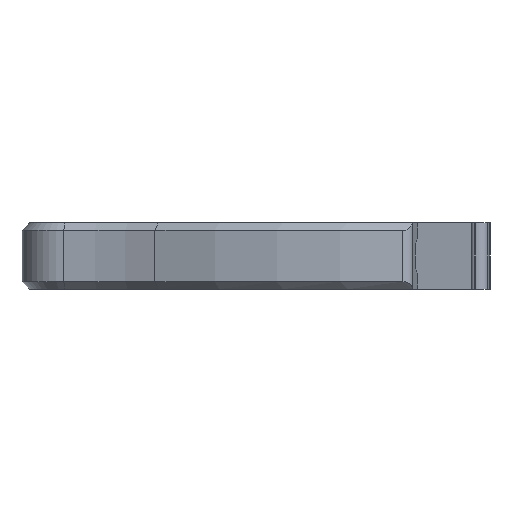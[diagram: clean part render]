
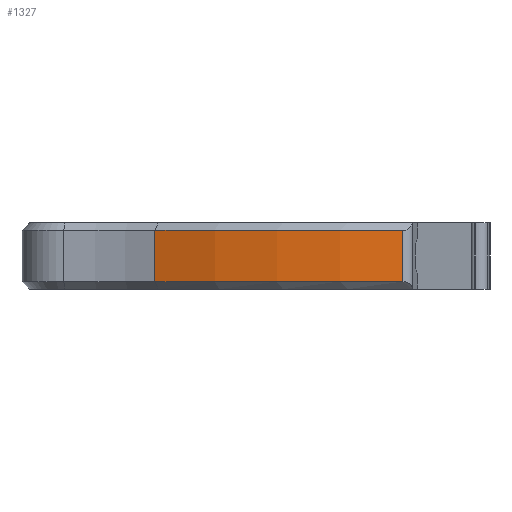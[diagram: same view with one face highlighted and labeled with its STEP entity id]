
A CAD part, left-side view. The second image highlights one B-rep face of the part: STEP entity #1327.
In plain terms, the highlighted cylindrical face has radius 77.47 mm (diameter 154.94 mm), a partial arc.
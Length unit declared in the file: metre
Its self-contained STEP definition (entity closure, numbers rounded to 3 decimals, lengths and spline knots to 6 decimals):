
#32=CYLINDRICAL_SURFACE('',#1465,0.07747);
#113=CIRCLE('',#1466,0.07747);
#114=CIRCLE('',#1467,0.07747);
#321=ORIENTED_EDGE('',*,*,#669,.F.);
#322=ORIENTED_EDGE('',*,*,#670,.T.);
#323=ORIENTED_EDGE('',*,*,#666,.T.);
#324=ORIENTED_EDGE('',*,*,#671,.T.);
#666=EDGE_CURVE('',#832,#833,#937,.T.);
#669=EDGE_CURVE('',#834,#835,#938,.T.);
#670=EDGE_CURVE('',#834,#832,#113,.F.);
#671=EDGE_CURVE('',#833,#835,#114,.T.);
#832=VERTEX_POINT('',#2243);
#833=VERTEX_POINT('',#2244);
#834=VERTEX_POINT('',#2257);
#835=VERTEX_POINT('',#2258);
#937=LINE('',#2242,#1062);
#938=LINE('',#2256,#1063);
#1062=VECTOR('',#1767,1.);
#1063=VECTOR('',#1770,1.);
#1127=EDGE_LOOP('',(#321,#322,#323,#324));
#1211=FACE_BOUND('',#1127,.T.);
#1327=ADVANCED_FACE('',(#1211),#32,.T.);
#1465=AXIS2_PLACEMENT_3D('',#2255,#1768,#1769);
#1466=AXIS2_PLACEMENT_3D('',#2259,#1771,#1772);
#1467=AXIS2_PLACEMENT_3D('',#2260,#1773,#1774);
#1767=DIRECTION('',(0.,0.,1.));
#1768=DIRECTION('',(0.,0.,1.));
#1769=DIRECTION('',(1.,0.,0.));
#1770=DIRECTION('',(0.,0.,1.));
#1771=DIRECTION('',(0.,0.,-1.));
#1772=DIRECTION('',(-1.,0.,0.));
#1773=DIRECTION('',(0.,0.,-1.));
#1774=DIRECTION('',(-1.,0.,0.));
#2242=CARTESIAN_POINT('',(-0.070871,-0.010297,-0.010998));
#2243=CARTESIAN_POINT('',(-0.070871,-0.010297,-0.009728));
#2244=CARTESIAN_POINT('',(-0.070871,-0.010297,-0.00127));
#2255=CARTESIAN_POINT('',(0.005865,0.00034,-0.010998));
#2256=CARTESIAN_POINT('',(-0.065353,0.03083,-0.010998));
#2257=CARTESIAN_POINT('',(-0.065353,0.03083,-0.009728));
#2258=CARTESIAN_POINT('',(-0.065353,0.03083,-0.00127));
#2259=CARTESIAN_POINT('',(0.005865,0.00034,-0.009728));
#2260=CARTESIAN_POINT('',(0.005865,0.00034,-0.00127));
